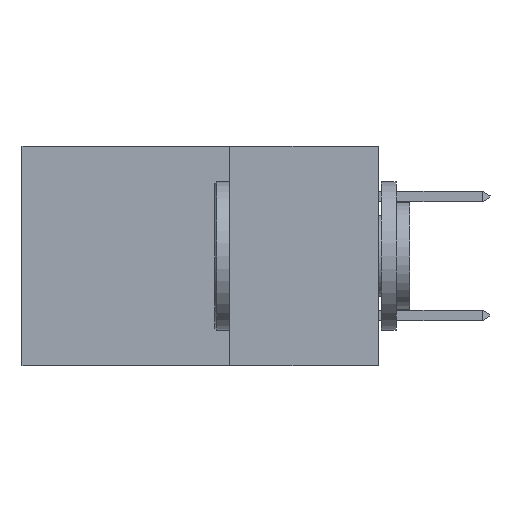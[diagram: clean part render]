
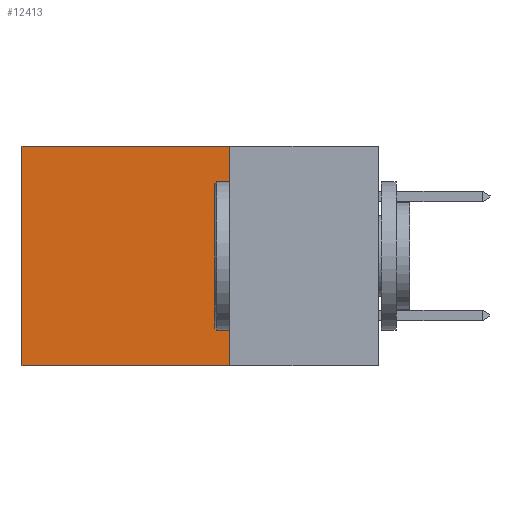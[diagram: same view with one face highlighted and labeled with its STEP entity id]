
A CAD part, left-side view. The second image highlights one B-rep face of the part: STEP entity #12413.
In plain terms, the highlighted planar face has unit normal (-1, 0, 0).
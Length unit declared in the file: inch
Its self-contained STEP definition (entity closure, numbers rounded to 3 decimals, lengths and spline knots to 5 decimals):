
#97 = DIRECTION ( 'NONE',  ( 0., 0., -1. ) ) ;
#403 = CARTESIAN_POINT ( 'NONE',  ( 0.2615, 0.25, -0.37 ) ) ;
#465 = EDGE_LOOP ( 'NONE', ( #15595, #9138, #6966, #875 ) ) ;
#584 = VERTEX_POINT ( 'NONE', #8479 ) ;
#875 = ORIENTED_EDGE ( 'NONE', *, *, #17638, .T. ) ;
#1330 = DIRECTION ( 'NONE',  ( 0., 1., 0. ) ) ;
#2413 = DIRECTION ( 'NONE',  ( 0., 1., 0. ) ) ;
#2586 = CARTESIAN_POINT ( 'NONE',  ( 0.2615, 0.6, -0.37 ) ) ;
#2912 = VERTEX_POINT ( 'NONE', #8101 ) ;
#6382 = PLANE ( 'NONE',  #13700 ) ;
#6966 = ORIENTED_EDGE ( 'NONE', *, *, #10735, .F. ) ;
#7131 = LINE ( 'NONE', #15838, #12436 ) ;
#7635 = DIRECTION ( 'NONE',  ( 1., 0., 0. ) ) ;
#8101 = CARTESIAN_POINT ( 'NONE',  ( 0.2615, 0.25, 0. ) ) ;
#8479 = CARTESIAN_POINT ( 'NONE',  ( 0.2615, 0.6, 0. ) ) ;
#8820 = CARTESIAN_POINT ( 'NONE',  ( 0.2615, 0.25, -0.37 ) ) ;
#9138 = ORIENTED_EDGE ( 'NONE', *, *, #14456, .F. ) ;
#9522 = VERTEX_POINT ( 'NONE', #12535 ) ;
#10268 = LINE ( 'NONE', #8820, #15511 ) ;
#10735 = EDGE_CURVE ( 'NONE', #2912, #9522, #10268, .T. ) ;
#11912 = VECTOR ( 'NONE', #97, 39.37008 ) ;
#12413 = ADVANCED_FACE ( 'NONE', ( #15099 ), #6382, .F. ) ;
#12436 = VECTOR ( 'NONE', #2413, 39.37008 ) ;
#12535 = CARTESIAN_POINT ( 'NONE',  ( 0.2615, 0.25, -0.37 ) ) ;
#13312 = LINE ( 'NONE', #14688, #11912 ) ;
#13700 = AXIS2_PLACEMENT_3D ( 'NONE', #403, #7635, #17891 ) ;
#14079 = EDGE_CURVE ( 'NONE', #584, #18947, #13312, .T. ) ;
#14456 = EDGE_CURVE ( 'NONE', #9522, #18947, #18445, .T. ) ;
#14688 = CARTESIAN_POINT ( 'NONE',  ( 0.2615, 0.6, -0.37 ) ) ;
#15099 = FACE_OUTER_BOUND ( 'NONE', #465, .T. ) ;
#15352 = VECTOR ( 'NONE', #1330, 39.37008 ) ;
#15511 = VECTOR ( 'NONE', #17445, 39.37008 ) ;
#15595 = ORIENTED_EDGE ( 'NONE', *, *, #14079, .T. ) ;
#15838 = CARTESIAN_POINT ( 'NONE',  ( 0.2615, 0.25, 0. ) ) ;
#17445 = DIRECTION ( 'NONE',  ( 0., 0., -1. ) ) ;
#17575 = CARTESIAN_POINT ( 'NONE',  ( 0.2615, 0.25, -0.37 ) ) ;
#17638 = EDGE_CURVE ( 'NONE', #2912, #584, #7131, .T. ) ;
#17891 = DIRECTION ( 'NONE',  ( 0., 0., -1. ) ) ;
#18445 = LINE ( 'NONE', #17575, #15352 ) ;
#18947 = VERTEX_POINT ( 'NONE', #2586 ) ;
